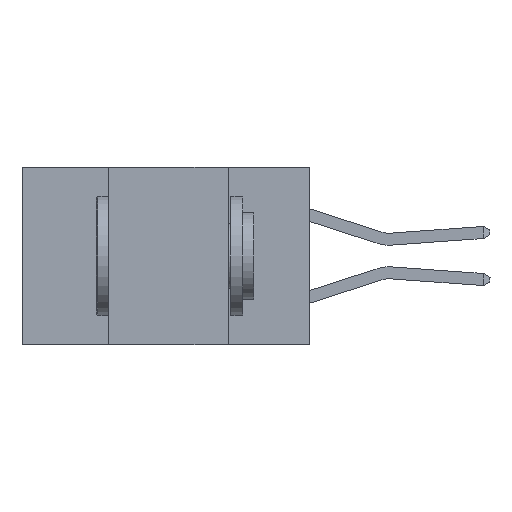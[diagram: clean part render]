
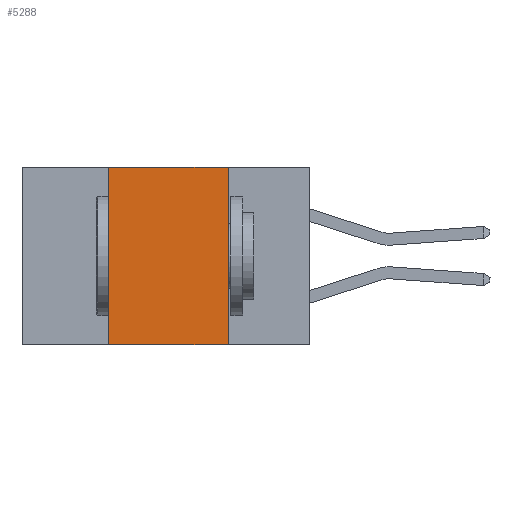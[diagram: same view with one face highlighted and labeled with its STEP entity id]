
A CAD part, left-side view. The second image highlights one B-rep face of the part: STEP entity #5288.
In plain terms, the highlighted planar face has unit normal (-1, 0, 0).
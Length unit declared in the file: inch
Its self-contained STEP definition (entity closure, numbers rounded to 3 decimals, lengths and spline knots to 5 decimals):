
#272 = VERTEX_POINT ( 'NONE', #6318 ) ;
#466 = EDGE_LOOP ( 'NONE', ( #15228, #6586, #16421, #9945 ) ) ;
#1122 = EDGE_CURVE ( 'NONE', #6531, #15354, #17514, .T. ) ;
#1301 = FACE_OUTER_BOUND ( 'NONE', #466, .T. ) ;
#1899 = DIRECTION ( 'NONE',  ( 0., 0., -1. ) ) ;
#2839 = DIRECTION ( 'NONE',  ( 0., -1., 0. ) ) ;
#3033 = CARTESIAN_POINT ( 'NONE',  ( 0., 0.6, 0. ) ) ;
#3330 = VECTOR ( 'NONE', #5228, 39.37008 ) ;
#3772 = VECTOR ( 'NONE', #2839, 39.37008 ) ;
#4381 = VECTOR ( 'NONE', #10800, 39.37008 ) ;
#5228 = DIRECTION ( 'NONE',  ( 0., 0., 1. ) ) ;
#5288 = ADVANCED_FACE ( 'NONE', ( #1301 ), #8150, .F. ) ;
#6318 = CARTESIAN_POINT ( 'NONE',  ( 0., 0.17, 0. ) ) ;
#6531 = VERTEX_POINT ( 'NONE', #15824 ) ;
#6586 = ORIENTED_EDGE ( 'NONE', *, *, #12127, .F. ) ;
#7809 = CARTESIAN_POINT ( 'NONE',  ( 0., 0.42, 0. ) ) ;
#8150 = PLANE ( 'NONE',  #10413 ) ;
#8201 = DIRECTION ( 'NONE',  ( 1., 0., 0. ) ) ;
#9945 = ORIENTED_EDGE ( 'NONE', *, *, #1122, .T. ) ;
#10282 = DIRECTION ( 'NONE',  ( 0., -1., 0. ) ) ;
#10413 = AXIS2_PLACEMENT_3D ( 'NONE', #11083, #8201, #1899 ) ;
#10711 = EDGE_CURVE ( 'NONE', #6531, #18364, #18683, .T. ) ;
#10800 = DIRECTION ( 'NONE',  ( 0., 0., -1. ) ) ;
#11083 = CARTESIAN_POINT ( 'NONE',  ( 0., 0.6, 0. ) ) ;
#12127 = EDGE_CURVE ( 'NONE', #18364, #272, #17675, .T. ) ;
#13223 = VECTOR ( 'NONE', #10282, 39.37008 ) ;
#14077 = CARTESIAN_POINT ( 'NONE',  ( 0., 0.17, 0. ) ) ;
#14278 = CARTESIAN_POINT ( 'NONE',  ( 0., 0.17, -0.37 ) ) ;
#15228 = ORIENTED_EDGE ( 'NONE', *, *, #17287, .F. ) ;
#15354 = VERTEX_POINT ( 'NONE', #14278 ) ;
#15362 = LINE ( 'NONE', #14077, #4381 ) ;
#15824 = CARTESIAN_POINT ( 'NONE',  ( 0., 0.42, -0.37 ) ) ;
#15982 = CARTESIAN_POINT ( 'NONE',  ( 0., 0.42, 0. ) ) ;
#16421 = ORIENTED_EDGE ( 'NONE', *, *, #10711, .F. ) ;
#17287 = EDGE_CURVE ( 'NONE', #272, #15354, #15362, .T. ) ;
#17514 = LINE ( 'NONE', #19479, #13223 ) ;
#17675 = LINE ( 'NONE', #3033, #3772 ) ;
#18364 = VERTEX_POINT ( 'NONE', #15982 ) ;
#18683 = LINE ( 'NONE', #7809, #3330 ) ;
#19479 = CARTESIAN_POINT ( 'NONE',  ( 0., 0.6, -0.37 ) ) ;
